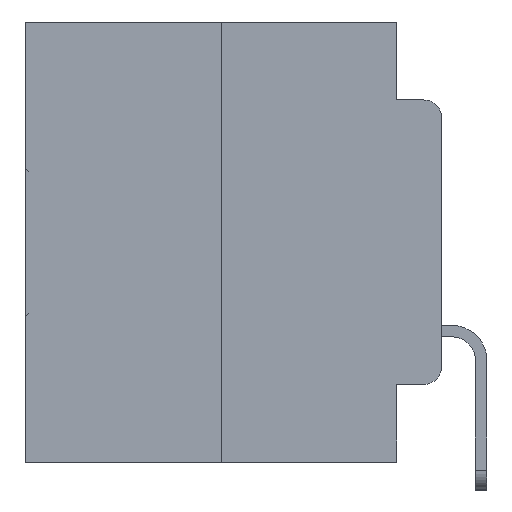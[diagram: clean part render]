
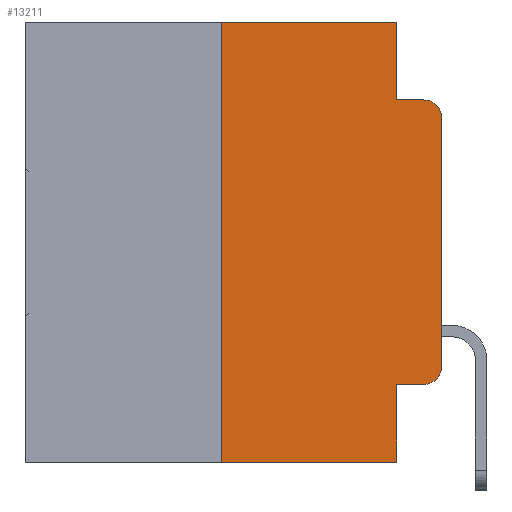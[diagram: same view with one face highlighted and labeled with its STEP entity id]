
A CAD part, left-side view. The second image highlights one B-rep face of the part: STEP entity #13211.
In plain terms, the highlighted planar face has unit normal (-1, 0, 0).
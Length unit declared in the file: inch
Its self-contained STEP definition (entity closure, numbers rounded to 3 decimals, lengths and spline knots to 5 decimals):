
#180 = VECTOR ( 'NONE', #5954, 39.37008 ) ;
#887 = CARTESIAN_POINT ( 'NONE',  ( 0., 0.02, -0.0885 ) ) ;
#975 = EDGE_CURVE ( 'NONE', #4082, #28676, #12172, .T. ) ;
#1678 = EDGE_CURVE ( 'NONE', #30154, #29927, #15638, .T. ) ;
#1686 = LINE ( 'NONE', #9993, #14345 ) ;
#2000 = PLANE ( 'NONE',  #22552 ) ;
#2649 = CARTESIAN_POINT ( 'NONE',  ( 0., 0., -0.1085 ) ) ;
#2771 = ORIENTED_EDGE ( 'NONE', *, *, #975, .F. ) ;
#3186 = CARTESIAN_POINT ( 'NONE',  ( 0., 0.051, -0.5 ) ) ;
#3821 = CARTESIAN_POINT ( 'NONE',  ( 0., 0.25, 0. ) ) ;
#4082 = VERTEX_POINT ( 'NONE', #20342 ) ;
#4597 = CARTESIAN_POINT ( 'NONE',  ( 0., 0.473, 0. ) ) ;
#4812 = ORIENTED_EDGE ( 'NONE', *, *, #9536, .F. ) ;
#5143 = EDGE_CURVE ( 'NONE', #29927, #9505, #17106, .T. ) ;
#5475 = CARTESIAN_POINT ( 'NONE',  ( 0., 0.02, -0.3915 ) ) ;
#5618 = ORIENTED_EDGE ( 'NONE', *, *, #14590, .T. ) ;
#5954 = DIRECTION ( 'NONE',  ( 0., -1., 0. ) ) ;
#6111 = CARTESIAN_POINT ( 'NONE',  ( 0., 0., -0.3915 ) ) ;
#6128 = DIRECTION ( 'NONE',  ( 0., 0., -1. ) ) ;
#6210 = EDGE_CURVE ( 'NONE', #25363, #6945, #14078, .T. ) ;
#6726 = LINE ( 'NONE', #8657, #30493 ) ;
#6782 = ORIENTED_EDGE ( 'NONE', *, *, #6210, .F. ) ;
#6888 = AXIS2_PLACEMENT_3D ( 'NONE', #23599, #9136, #25919 ) ;
#6945 = VERTEX_POINT ( 'NONE', #3821 ) ;
#7062 = LINE ( 'NONE', #15820, #180 ) ;
#7143 = DIRECTION ( 'NONE',  ( 1., 0., 0. ) ) ;
#7327 = EDGE_LOOP ( 'NONE', ( #29532, #24930, #21616, #2771, #11045, #6782, #15708, #4812, #5618, #25686 ) ) ;
#7422 = VECTOR ( 'NONE', #16261, 39.37008 ) ;
#8042 = DIRECTION ( 'NONE',  ( 0., 0., -1. ) ) ;
#8227 = LINE ( 'NONE', #15848, #26625 ) ;
#8657 = CARTESIAN_POINT ( 'NONE',  ( 0., 0.051, 0. ) ) ;
#9136 = DIRECTION ( 'NONE',  ( -1., 0., 0. ) ) ;
#9505 = VERTEX_POINT ( 'NONE', #887 ) ;
#9536 = EDGE_CURVE ( 'NONE', #22633, #12424, #6726, .T. ) ;
#9882 = CARTESIAN_POINT ( 'NONE',  ( 0., 0.473, -0.5 ) ) ;
#9993 = CARTESIAN_POINT ( 'NONE',  ( 0., 0.051, -0.4115 ) ) ;
#10389 = DIRECTION ( 'NONE',  ( 0., 0., -1. ) ) ;
#11045 = ORIENTED_EDGE ( 'NONE', *, *, #18581, .F. ) ;
#12172 = LINE ( 'NONE', #27102, #17114 ) ;
#12415 = DIRECTION ( 'NONE',  ( 0., -1., 0. ) ) ;
#12424 = VERTEX_POINT ( 'NONE', #3186 ) ;
#13084 = CIRCLE ( 'NONE', #14191, 0.02 ) ;
#13211 = ADVANCED_FACE ( 'NONE', ( #30948 ), #2000, .F. ) ;
#13316 = CARTESIAN_POINT ( 'NONE',  ( 0., 0.051, -0.0885 ) ) ;
#14078 = LINE ( 'NONE', #30139, #7422 ) ;
#14191 = AXIS2_PLACEMENT_3D ( 'NONE', #5475, #22516, #8042 ) ;
#14345 = VECTOR ( 'NONE', #29005, 39.37008 ) ;
#14590 = EDGE_CURVE ( 'NONE', #22633, #19339, #1686, .T. ) ;
#15638 = LINE ( 'NONE', #27651, #26699 ) ;
#15708 = ORIENTED_EDGE ( 'NONE', *, *, #21868, .T. ) ;
#15820 = CARTESIAN_POINT ( 'NONE',  ( 0., 0.473, 0. ) ) ;
#15848 = CARTESIAN_POINT ( 'NONE',  ( 0., 0.051, -0.0885 ) ) ;
#16261 = DIRECTION ( 'NONE',  ( 0., 0., 1. ) ) ;
#17106 = CIRCLE ( 'NONE', #6888, 0.02 ) ;
#17114 = VECTOR ( 'NONE', #10389, 39.37008 ) ;
#17753 = CARTESIAN_POINT ( 'NONE',  ( 0., 0.02, -0.4115 ) ) ;
#18581 = EDGE_CURVE ( 'NONE', #6945, #4082, #7062, .T. ) ;
#19330 = EDGE_CURVE ( 'NONE', #19339, #30154, #13084, .T. ) ;
#19339 = VERTEX_POINT ( 'NONE', #17753 ) ;
#20342 = CARTESIAN_POINT ( 'NONE',  ( 0., 0.051, 0. ) ) ;
#21504 = EDGE_CURVE ( 'NONE', #28676, #9505, #8227, .T. ) ;
#21616 = ORIENTED_EDGE ( 'NONE', *, *, #21504, .F. ) ;
#21868 = EDGE_CURVE ( 'NONE', #25363, #12424, #29392, .T. ) ;
#22516 = DIRECTION ( 'NONE',  ( -1., 0., 0. ) ) ;
#22552 = AXIS2_PLACEMENT_3D ( 'NONE', #4597, #7143, #24080 ) ;
#22633 = VERTEX_POINT ( 'NONE', #30604 ) ;
#23599 = CARTESIAN_POINT ( 'NONE',  ( 0., 0.02, -0.1085 ) ) ;
#24080 = DIRECTION ( 'NONE',  ( 0., 0., -1. ) ) ;
#24930 = ORIENTED_EDGE ( 'NONE', *, *, #5143, .T. ) ;
#25360 = DIRECTION ( 'NONE',  ( 0., -1., 0. ) ) ;
#25363 = VERTEX_POINT ( 'NONE', #29716 ) ;
#25686 = ORIENTED_EDGE ( 'NONE', *, *, #19330, .T. ) ;
#25919 = DIRECTION ( 'NONE',  ( 0., 0., -1. ) ) ;
#26625 = VECTOR ( 'NONE', #25360, 39.37008 ) ;
#26699 = VECTOR ( 'NONE', #27742, 39.37008 ) ;
#27102 = CARTESIAN_POINT ( 'NONE',  ( 0., 0.051, 0. ) ) ;
#27651 = CARTESIAN_POINT ( 'NONE',  ( 0., 0., 0. ) ) ;
#27742 = DIRECTION ( 'NONE',  ( 0., 0., 1. ) ) ;
#28676 = VERTEX_POINT ( 'NONE', #13316 ) ;
#28712 = VECTOR ( 'NONE', #12415, 39.37008 ) ;
#29005 = DIRECTION ( 'NONE',  ( 0., -1., 0. ) ) ;
#29392 = LINE ( 'NONE', #9882, #28712 ) ;
#29532 = ORIENTED_EDGE ( 'NONE', *, *, #1678, .T. ) ;
#29716 = CARTESIAN_POINT ( 'NONE',  ( 0., 0.25, -0.5 ) ) ;
#29927 = VERTEX_POINT ( 'NONE', #2649 ) ;
#30139 = CARTESIAN_POINT ( 'NONE',  ( 0., 0.25, 0. ) ) ;
#30154 = VERTEX_POINT ( 'NONE', #6111 ) ;
#30493 = VECTOR ( 'NONE', #6128, 39.37008 ) ;
#30604 = CARTESIAN_POINT ( 'NONE',  ( 0., 0.051, -0.4115 ) ) ;
#30948 = FACE_OUTER_BOUND ( 'NONE', #7327, .T. ) ;
